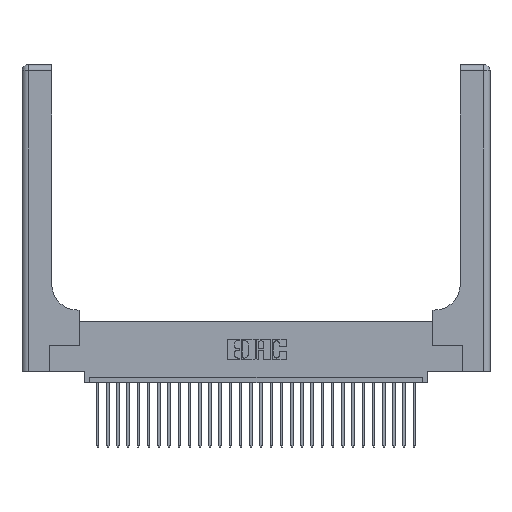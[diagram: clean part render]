
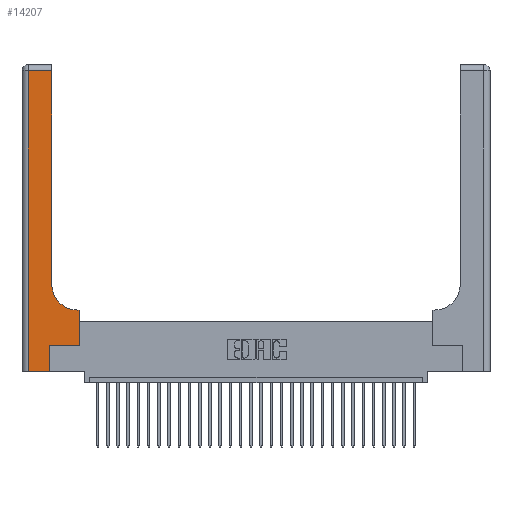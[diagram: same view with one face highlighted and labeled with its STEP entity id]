
A CAD part, top view. The second image highlights one B-rep face of the part: STEP entity #14207.
In plain terms, the highlighted planar face has unit normal (0, 0, 1).
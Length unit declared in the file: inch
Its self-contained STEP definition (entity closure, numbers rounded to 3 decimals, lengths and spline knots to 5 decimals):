
#5 = VERTEX_POINT ( 'NONE', #1311 ) ;
#209 = LINE ( 'NONE', #29825, #24731 ) ;
#376 = DIRECTION ( 'NONE',  ( 0., -1., 0. ) ) ;
#1311 = CARTESIAN_POINT ( 'NONE',  ( 0.5415, 0.6, 0.37 ) ) ;
#1493 = DIRECTION ( 'NONE',  ( -1., 0., 0. ) ) ;
#1710 = CARTESIAN_POINT ( 'NONE',  ( 0.269, 0.25, 0.37 ) ) ;
#2108 = PLANE ( 'NONE',  #4364 ) ;
#2249 = LINE ( 'NONE', #7537, #27537 ) ;
#2494 = VERTEX_POINT ( 'NONE', #13817 ) ;
#2657 = CARTESIAN_POINT ( 'NONE',  ( 0.06, 0., 0.37 ) ) ;
#3047 = VERTEX_POINT ( 'NONE', #5014 ) ;
#3420 = CIRCLE ( 'NONE', #13149, 0.25 ) ;
#3623 = FACE_OUTER_BOUND ( 'NONE', #16717, .T. ) ;
#4364 = AXIS2_PLACEMENT_3D ( 'NONE', #4479, #25907, #21718 ) ;
#4479 = CARTESIAN_POINT ( 'NONE',  ( 0., 3., 0.37 ) ) ;
#4717 = VERTEX_POINT ( 'NONE', #2657 ) ;
#4946 = EDGE_CURVE ( 'NONE', #13095, #7128, #12320, .T. ) ;
#5014 = CARTESIAN_POINT ( 'NONE',  ( 0.06, 2.94, 0.37 ) ) ;
#5046 = DIRECTION ( 'NONE',  ( 0., 1., 0. ) ) ;
#5545 = EDGE_CURVE ( 'NONE', #4717, #2494, #2249, .T. ) ;
#6036 = ORIENTED_EDGE ( 'NONE', *, *, #4946, .T. ) ;
#7128 = VERTEX_POINT ( 'NONE', #27627 ) ;
#7537 = CARTESIAN_POINT ( 'NONE',  ( 0., 0., 0.37 ) ) ;
#8318 = EDGE_CURVE ( 'NONE', #15749, #3047, #10300, .T. ) ;
#8689 = ORIENTED_EDGE ( 'NONE', *, *, #27863, .T. ) ;
#8962 = LINE ( 'NONE', #19250, #19320 ) ;
#8965 = ORIENTED_EDGE ( 'NONE', *, *, #18515, .T. ) ;
#9229 = EDGE_CURVE ( 'NONE', #2494, #13095, #209, .T. ) ;
#9356 = ORIENTED_EDGE ( 'NONE', *, *, #18614, .T. ) ;
#10251 = VERTEX_POINT ( 'NONE', #26077 ) ;
#10300 = LINE ( 'NONE', #23509, #24014 ) ;
#12320 = LINE ( 'NONE', #25589, #29433 ) ;
#12562 = DIRECTION ( 'NONE',  ( 0., 0., -1. ) ) ;
#12625 = CARTESIAN_POINT ( 'NONE',  ( 0.2915, 0.85, 0.37 ) ) ;
#12950 = EDGE_CURVE ( 'NONE', #10251, #5, #20030, .T. ) ;
#13095 = VERTEX_POINT ( 'NONE', #1710 ) ;
#13149 = AXIS2_PLACEMENT_3D ( 'NONE', #15177, #12562, #19826 ) ;
#13422 = LINE ( 'NONE', #19042, #26440 ) ;
#13780 = CARTESIAN_POINT ( 'NONE',  ( 0.5585, 0.25, 0.37 ) ) ;
#13817 = CARTESIAN_POINT ( 'NONE',  ( 0.269, 0., 0.37 ) ) ;
#14207 = ADVANCED_FACE ( 'NONE', ( #3623 ), #2108, .F. ) ;
#15177 = CARTESIAN_POINT ( 'NONE',  ( 0.5415, 0.85, 0.37 ) ) ;
#15749 = VERTEX_POINT ( 'NONE', #29381 ) ;
#16155 = DIRECTION ( 'NONE',  ( -1., 0., 0. ) ) ;
#16159 = DIRECTION ( 'NONE',  ( 0., 1., 0. ) ) ;
#16691 = VECTOR ( 'NONE', #1493, 39.37008 ) ;
#16717 = EDGE_LOOP ( 'NONE', ( #8965, #17148, #9356, #24799, #19346, #6036, #30382, #20203, #8689 ) ) ;
#17148 = ORIENTED_EDGE ( 'NONE', *, *, #8318, .T. ) ;
#17229 = VECTOR ( 'NONE', #16159, 39.37008 ) ;
#17902 = CARTESIAN_POINT ( 'NONE',  ( 0.2915, 0.6, 0.37 ) ) ;
#18515 = EDGE_CURVE ( 'NONE', #26276, #15749, #13422, .T. ) ;
#18614 = EDGE_CURVE ( 'NONE', #3047, #4717, #8962, .T. ) ;
#19042 = CARTESIAN_POINT ( 'NONE',  ( 0.2915, 3., 0.37 ) ) ;
#19250 = CARTESIAN_POINT ( 'NONE',  ( 0.06, 3., 0.37 ) ) ;
#19320 = VECTOR ( 'NONE', #376, 39.37008 ) ;
#19346 = ORIENTED_EDGE ( 'NONE', *, *, #9229, .T. ) ;
#19826 = DIRECTION ( 'NONE',  ( 1., 0., 0. ) ) ;
#20030 = LINE ( 'NONE', #17902, #16691 ) ;
#20203 = ORIENTED_EDGE ( 'NONE', *, *, #12950, .T. ) ;
#21718 = DIRECTION ( 'NONE',  ( -1., 0., 0. ) ) ;
#21720 = DIRECTION ( 'NONE',  ( 1., 0., 0. ) ) ;
#23509 = CARTESIAN_POINT ( 'NONE',  ( 0., 2.94, 0.37 ) ) ;
#24014 = VECTOR ( 'NONE', #16155, 39.37008 ) ;
#24731 = VECTOR ( 'NONE', #25058, 39.37008 ) ;
#24799 = ORIENTED_EDGE ( 'NONE', *, *, #5545, .T. ) ;
#25058 = DIRECTION ( 'NONE',  ( 0., 1., 0. ) ) ;
#25065 = LINE ( 'NONE', #13780, #17229 ) ;
#25589 = CARTESIAN_POINT ( 'NONE',  ( 0.269, 0.25, 0.37 ) ) ;
#25907 = DIRECTION ( 'NONE',  ( 0., 0., -1. ) ) ;
#26077 = CARTESIAN_POINT ( 'NONE',  ( 0.5585, 0.6, 0.37 ) ) ;
#26276 = VERTEX_POINT ( 'NONE', #12625 ) ;
#26440 = VECTOR ( 'NONE', #5046, 39.37008 ) ;
#26590 = EDGE_CURVE ( 'NONE', #7128, #10251, #25065, .T. ) ;
#27537 = VECTOR ( 'NONE', #21720, 39.37008 ) ;
#27627 = CARTESIAN_POINT ( 'NONE',  ( 0.5585, 0.25, 0.37 ) ) ;
#27863 = EDGE_CURVE ( 'NONE', #5, #26276, #3420, .T. ) ;
#28076 = DIRECTION ( 'NONE',  ( 1., 0., 0. ) ) ;
#29381 = CARTESIAN_POINT ( 'NONE',  ( 0.2915, 2.94, 0.37 ) ) ;
#29433 = VECTOR ( 'NONE', #28076, 39.37008 ) ;
#29825 = CARTESIAN_POINT ( 'NONE',  ( 0.269, 0., 0.37 ) ) ;
#30382 = ORIENTED_EDGE ( 'NONE', *, *, #26590, .T. ) ;
